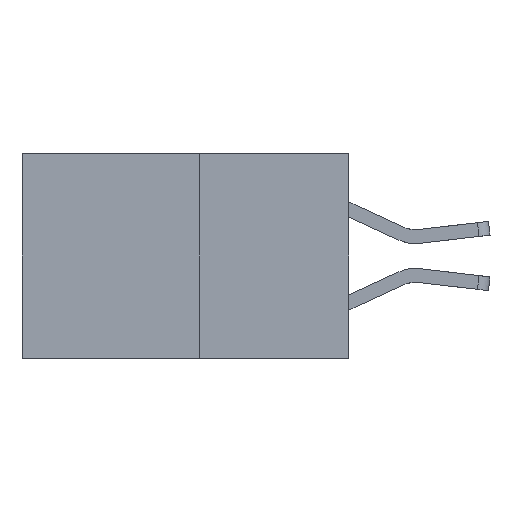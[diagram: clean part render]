
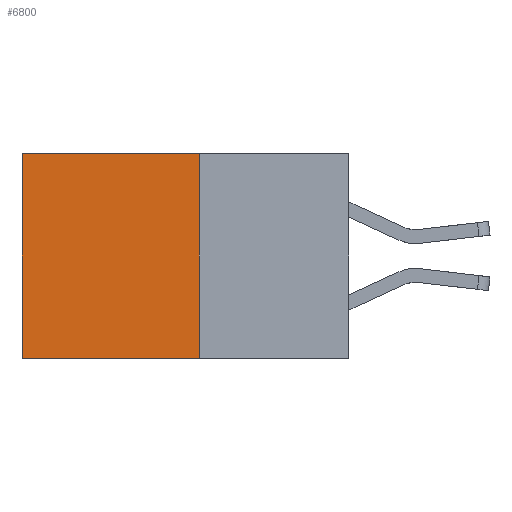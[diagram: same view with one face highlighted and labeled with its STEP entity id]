
A CAD part, left-side view. The second image highlights one B-rep face of the part: STEP entity #6800.
In plain terms, the highlighted planar face has unit normal (-1, 0, 0).
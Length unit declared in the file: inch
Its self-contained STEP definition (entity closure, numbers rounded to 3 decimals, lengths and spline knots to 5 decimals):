
#35 = EDGE_CURVE ( 'NONE', #7166, #6504, #6757, .T. ) ;
#61 = VECTOR ( 'NONE', #512, 39.37008 ) ;
#426 = EDGE_CURVE ( 'NONE', #8005, #8046, #7262, .T. ) ;
#512 = DIRECTION ( 'NONE',  ( 0., 0., -1. ) ) ;
#733 = DIRECTION ( 'NONE',  ( 0., 1., 0. ) ) ;
#1582 = PLANE ( 'NONE',  #6161 ) ;
#1813 = EDGE_CURVE ( 'NONE', #8046, #6504, #5664, .T. ) ;
#2083 = DIRECTION ( 'NONE',  ( 0., 1., 0. ) ) ;
#2554 = ORIENTED_EDGE ( 'NONE', *, *, #9479, .F. ) ;
#3097 = CARTESIAN_POINT ( 'NONE',  ( 0.277, 0.27, -0.37 ) ) ;
#3124 = ORIENTED_EDGE ( 'NONE', *, *, #1813, .T. ) ;
#3459 = CARTESIAN_POINT ( 'NONE',  ( 0.277, 0.27, -0.37 ) ) ;
#3926 = CARTESIAN_POINT ( 'NONE',  ( 0.277, 0.59, -0.37 ) ) ;
#4303 = VECTOR ( 'NONE', #733, 39.37008 ) ;
#4347 = DIRECTION ( 'NONE',  ( 0., 0., -1. ) ) ;
#4649 = FACE_OUTER_BOUND ( 'NONE', #10665, .T. ) ;
#4848 = ORIENTED_EDGE ( 'NONE', *, *, #426, .T. ) ;
#4997 = LINE ( 'NONE', #9770, #61 ) ;
#5099 = ORIENTED_EDGE ( 'NONE', *, *, #35, .F. ) ;
#5251 = CARTESIAN_POINT ( 'NONE',  ( 0.277, 0.27, -0.37 ) ) ;
#5664 = LINE ( 'NONE', #5942, #7609 ) ;
#5940 = DIRECTION ( 'NONE',  ( 0., 0., -1. ) ) ;
#5942 = CARTESIAN_POINT ( 'NONE',  ( 0.277, 0.59, -0.37 ) ) ;
#6161 = AXIS2_PLACEMENT_3D ( 'NONE', #3459, #9251, #4347 ) ;
#6504 = VERTEX_POINT ( 'NONE', #3926 ) ;
#6757 = LINE ( 'NONE', #5251, #4303 ) ;
#6800 = ADVANCED_FACE ( 'NONE', ( #4649 ), #1582, .F. ) ;
#7166 = VERTEX_POINT ( 'NONE', #3097 ) ;
#7262 = LINE ( 'NONE', #9570, #9187 ) ;
#7388 = CARTESIAN_POINT ( 'NONE',  ( 0.277, 0.59, 0. ) ) ;
#7609 = VECTOR ( 'NONE', #5940, 39.37008 ) ;
#8005 = VERTEX_POINT ( 'NONE', #8236 ) ;
#8046 = VERTEX_POINT ( 'NONE', #7388 ) ;
#8236 = CARTESIAN_POINT ( 'NONE',  ( 0.277, 0.27, 0. ) ) ;
#9187 = VECTOR ( 'NONE', #2083, 39.37008 ) ;
#9251 = DIRECTION ( 'NONE',  ( 1., 0., 0. ) ) ;
#9479 = EDGE_CURVE ( 'NONE', #8005, #7166, #4997, .T. ) ;
#9570 = CARTESIAN_POINT ( 'NONE',  ( 0.277, 0.27, 0. ) ) ;
#9770 = CARTESIAN_POINT ( 'NONE',  ( 0.277, 0.27, -0.37 ) ) ;
#10665 = EDGE_LOOP ( 'NONE', ( #3124, #5099, #2554, #4848 ) ) ;
